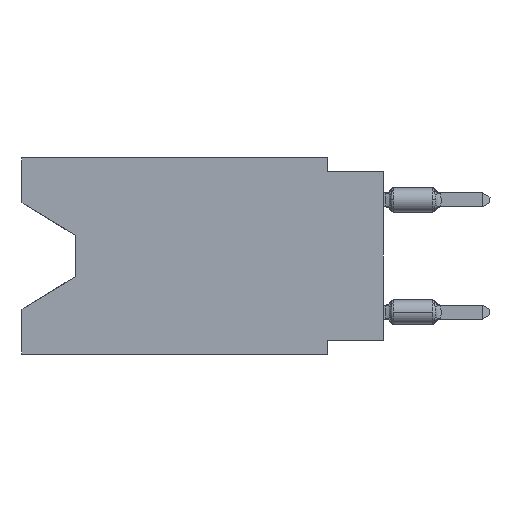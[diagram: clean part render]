
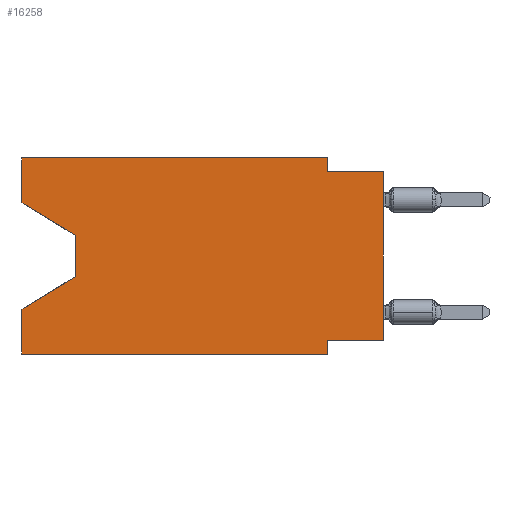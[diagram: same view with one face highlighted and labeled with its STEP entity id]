
A CAD part, left-side view. The second image highlights one B-rep face of the part: STEP entity #16258.
In plain terms, the highlighted planar face has unit normal (-1, 0, 0).
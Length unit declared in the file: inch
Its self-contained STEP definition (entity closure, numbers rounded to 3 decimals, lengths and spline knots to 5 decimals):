
#241 = DIRECTION ( 'NONE',  ( 0., 0., 1. ) ) ;
#599 = CARTESIAN_POINT ( 'NONE',  ( 0., 0.645, -0.08025 ) ) ;
#650 = EDGE_CURVE ( 'NONE', #13677, #4878, #7298, .T. ) ;
#1070 = EDGE_CURVE ( 'NONE', #22790, #9029, #3762, .T. ) ;
#2178 = DIRECTION ( 'NONE',  ( 0., -1., 0. ) ) ;
#2594 = CARTESIAN_POINT ( 'NONE',  ( 0., 0.55, -0.212 ) ) ;
#2890 = LINE ( 'NONE', #21649, #6944 ) ;
#2910 = ORIENTED_EDGE ( 'NONE', *, *, #13704, .T. ) ;
#3197 = LINE ( 'NONE', #15365, #4960 ) ;
#3253 = ORIENTED_EDGE ( 'NONE', *, *, #4290, .T. ) ;
#3330 = VECTOR ( 'NONE', #19019, 39.37008 ) ;
#3598 = CARTESIAN_POINT ( 'NONE',  ( 0., 0., -0.325 ) ) ;
#3762 = LINE ( 'NONE', #11369, #3330 ) ;
#3791 = CARTESIAN_POINT ( 'NONE',  ( 0., 0.55, -0.138 ) ) ;
#4028 = DIRECTION ( 'NONE',  ( 0., 0., -1. ) ) ;
#4120 = VECTOR ( 'NONE', #2178, 39.37008 ) ;
#4172 = PLANE ( 'NONE',  #7326 ) ;
#4231 = EDGE_CURVE ( 'NONE', #13125, #19197, #18516, .T. ) ;
#4290 = EDGE_CURVE ( 'NONE', #4966, #13677, #24503, .T. ) ;
#4335 = EDGE_CURVE ( 'NONE', #10285, #24711, #16992, .T. ) ;
#4507 = LINE ( 'NONE', #17619, #21573 ) ;
#4878 = VERTEX_POINT ( 'NONE', #2594 ) ;
#4960 = VECTOR ( 'NONE', #22444, 39.37008 ) ;
#4966 = VERTEX_POINT ( 'NONE', #599 ) ;
#5015 = DIRECTION ( 'NONE',  ( 0., -1., 0. ) ) ;
#5241 = DIRECTION ( 'NONE',  ( 0., -0.855, -0.519 ) ) ;
#5276 = CARTESIAN_POINT ( 'NONE',  ( 0., 0.55, -0.138 ) ) ;
#6288 = FACE_OUTER_BOUND ( 'NONE', #9462, .T. ) ;
#6676 = DIRECTION ( 'NONE',  ( 0., 0., -1. ) ) ;
#6944 = VECTOR ( 'NONE', #16255, 39.37008 ) ;
#7298 = LINE ( 'NONE', #3791, #16815 ) ;
#7326 = AXIS2_PLACEMENT_3D ( 'NONE', #8558, #12295, #6676 ) ;
#7373 = CARTESIAN_POINT ( 'NONE',  ( 0., 0.645, -0.08025 ) ) ;
#7380 = CARTESIAN_POINT ( 'NONE',  ( 0., 0.1, 0. ) ) ;
#7668 = EDGE_CURVE ( 'NONE', #22790, #9124, #3197, .T. ) ;
#7807 = CARTESIAN_POINT ( 'NONE',  ( 0., 0., -0.025 ) ) ;
#7951 = LINE ( 'NONE', #15199, #13378 ) ;
#8274 = CARTESIAN_POINT ( 'NONE',  ( 0., 0.645, -0.35 ) ) ;
#8558 = CARTESIAN_POINT ( 'NONE',  ( 0., 0.645, 0. ) ) ;
#9029 = VERTEX_POINT ( 'NONE', #9950 ) ;
#9124 = VERTEX_POINT ( 'NONE', #14338 ) ;
#9174 = VECTOR ( 'NONE', #5015, 39.37008 ) ;
#9190 = VERTEX_POINT ( 'NONE', #9413 ) ;
#9413 = CARTESIAN_POINT ( 'NONE',  ( 0., 0.1, -0.025 ) ) ;
#9462 = EDGE_LOOP ( 'NONE', ( #3253, #18399, #2910, #13644, #10454, #24550, #17908, #23770, #17785, #24441, #17412, #11618 ) ) ;
#9588 = CARTESIAN_POINT ( 'NONE',  ( 0., 0., 0. ) ) ;
#9718 = DIRECTION ( 'NONE',  ( 0., 0., -1. ) ) ;
#9733 = LINE ( 'NONE', #11739, #15476 ) ;
#9950 = CARTESIAN_POINT ( 'NONE',  ( 0., 0.645, -0.26975 ) ) ;
#10091 = CARTESIAN_POINT ( 'NONE',  ( 0., 0.1, 0. ) ) ;
#10109 = VECTOR ( 'NONE', #9718, 39.37008 ) ;
#10285 = VERTEX_POINT ( 'NONE', #3598 ) ;
#10286 = EDGE_CURVE ( 'NONE', #4966, #13125, #7951, .T. ) ;
#10454 = ORIENTED_EDGE ( 'NONE', *, *, #7668, .T. ) ;
#11162 = VECTOR ( 'NONE', #241, 39.37008 ) ;
#11369 = CARTESIAN_POINT ( 'NONE',  ( 0., 0.645, 0. ) ) ;
#11586 = EDGE_CURVE ( 'NONE', #16401, #9124, #4507, .T. ) ;
#11618 = ORIENTED_EDGE ( 'NONE', *, *, #10286, .F. ) ;
#11739 = CARTESIAN_POINT ( 'NONE',  ( 0., 0.55, -0.212 ) ) ;
#12295 = DIRECTION ( 'NONE',  ( 1., 0., 0. ) ) ;
#13125 = VERTEX_POINT ( 'NONE', #14812 ) ;
#13378 = VECTOR ( 'NONE', #24718, 39.37008 ) ;
#13644 = ORIENTED_EDGE ( 'NONE', *, *, #1070, .F. ) ;
#13677 = VERTEX_POINT ( 'NONE', #5276 ) ;
#13704 = EDGE_CURVE ( 'NONE', #4878, #9029, #9733, .T. ) ;
#14338 = CARTESIAN_POINT ( 'NONE',  ( 0., 0.1, -0.35 ) ) ;
#14812 = CARTESIAN_POINT ( 'NONE',  ( 0., 0.645, 0. ) ) ;
#14854 = CARTESIAN_POINT ( 'NONE',  ( 0., 0.645, 0. ) ) ;
#15032 = CARTESIAN_POINT ( 'NONE',  ( 0., 0., -0.025 ) ) ;
#15199 = CARTESIAN_POINT ( 'NONE',  ( 0., 0.645, 0. ) ) ;
#15365 = CARTESIAN_POINT ( 'NONE',  ( 0., 0.645, -0.35 ) ) ;
#15476 = VECTOR ( 'NONE', #21269, 39.37008 ) ;
#16092 = EDGE_CURVE ( 'NONE', #9190, #24711, #22812, .T. ) ;
#16255 = DIRECTION ( 'NONE',  ( 0., 1., 0. ) ) ;
#16258 = ADVANCED_FACE ( 'NONE', ( #6288 ), #4172, .F. ) ;
#16401 = VERTEX_POINT ( 'NONE', #22393 ) ;
#16475 = EDGE_CURVE ( 'NONE', #19197, #9190, #20649, .T. ) ;
#16815 = VECTOR ( 'NONE', #4028, 39.37008 ) ;
#16992 = LINE ( 'NONE', #9588, #11162 ) ;
#17412 = ORIENTED_EDGE ( 'NONE', *, *, #4231, .F. ) ;
#17619 = CARTESIAN_POINT ( 'NONE',  ( 0., 0.1, -0.35 ) ) ;
#17785 = ORIENTED_EDGE ( 'NONE', *, *, #16092, .F. ) ;
#17908 = ORIENTED_EDGE ( 'NONE', *, *, #23181, .F. ) ;
#18399 = ORIENTED_EDGE ( 'NONE', *, *, #650, .T. ) ;
#18516 = LINE ( 'NONE', #14854, #9174 ) ;
#19019 = DIRECTION ( 'NONE',  ( 0., 0., 1. ) ) ;
#19197 = VERTEX_POINT ( 'NONE', #10091 ) ;
#19389 = DIRECTION ( 'NONE',  ( 0., 0., -1. ) ) ;
#20649 = LINE ( 'NONE', #7380, #10109 ) ;
#21269 = DIRECTION ( 'NONE',  ( 0., 0.855, -0.519 ) ) ;
#21573 = VECTOR ( 'NONE', #19389, 39.37008 ) ;
#21649 = CARTESIAN_POINT ( 'NONE',  ( 0., 0., -0.325 ) ) ;
#21970 = VECTOR ( 'NONE', #5241, 39.37008 ) ;
#22393 = CARTESIAN_POINT ( 'NONE',  ( 0., 0.1, -0.325 ) ) ;
#22444 = DIRECTION ( 'NONE',  ( 0., -1., 0. ) ) ;
#22790 = VERTEX_POINT ( 'NONE', #8274 ) ;
#22812 = LINE ( 'NONE', #15032, #4120 ) ;
#23181 = EDGE_CURVE ( 'NONE', #10285, #16401, #2890, .T. ) ;
#23770 = ORIENTED_EDGE ( 'NONE', *, *, #4335, .T. ) ;
#24441 = ORIENTED_EDGE ( 'NONE', *, *, #16475, .F. ) ;
#24503 = LINE ( 'NONE', #7373, #21970 ) ;
#24550 = ORIENTED_EDGE ( 'NONE', *, *, #11586, .F. ) ;
#24711 = VERTEX_POINT ( 'NONE', #7807 ) ;
#24718 = DIRECTION ( 'NONE',  ( 0., 0., 1. ) ) ;
